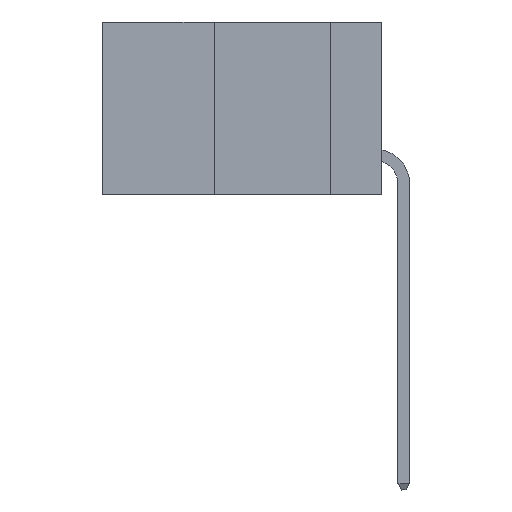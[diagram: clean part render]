
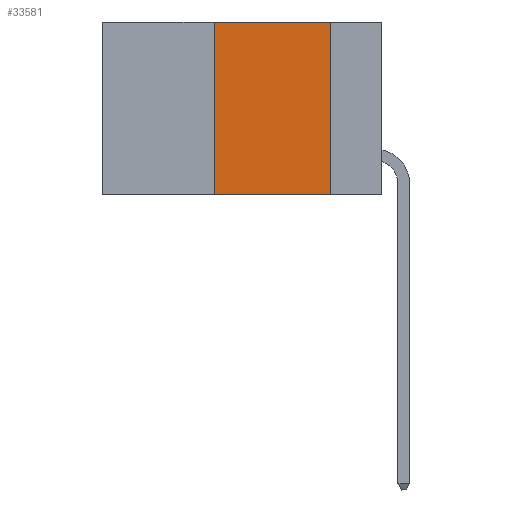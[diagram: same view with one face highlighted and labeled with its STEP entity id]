
A CAD part, left-side view. The second image highlights one B-rep face of the part: STEP entity #33581.
In plain terms, the highlighted planar face has unit normal (-1, 0, 0).
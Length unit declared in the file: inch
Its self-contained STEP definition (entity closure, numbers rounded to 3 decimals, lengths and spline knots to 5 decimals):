
#94 = VECTOR ( 'NONE', #6716, 39.37008 ) ;
#157 = VECTOR ( 'NONE', #35908, 39.37008 ) ;
#442 = ORIENTED_EDGE ( 'NONE', *, *, #18130, .F. ) ;
#4446 = ORIENTED_EDGE ( 'NONE', *, *, #7957, .T. ) ;
#4661 = EDGE_LOOP ( 'NONE', ( #442, #22245, #21265, #4446 ) ) ;
#6716 = DIRECTION ( 'NONE',  ( 0., 0., -1. ) ) ;
#7957 = EDGE_CURVE ( 'NONE', #26516, #17868, #40370, .T. ) ;
#8810 = PLANE ( 'NONE',  #37498 ) ;
#9765 = CARTESIAN_POINT ( 'NONE',  ( 0., 0.11, 0. ) ) ;
#10252 = EDGE_CURVE ( 'NONE', #26516, #10833, #16312, .T. ) ;
#10833 = VERTEX_POINT ( 'NONE', #28313 ) ;
#14839 = EDGE_CURVE ( 'NONE', #10833, #34850, #32149, .T. ) ;
#16312 = LINE ( 'NONE', #22886, #26755 ) ;
#16347 = DIRECTION ( 'NONE',  ( 0., 0., 1. ) ) ;
#16848 = CARTESIAN_POINT ( 'NONE',  ( 0., 0.6, 0. ) ) ;
#17218 = CARTESIAN_POINT ( 'NONE',  ( 0., 0.11, -0.37 ) ) ;
#17868 = VERTEX_POINT ( 'NONE', #17218 ) ;
#18130 = EDGE_CURVE ( 'NONE', #34850, #17868, #27435, .T. ) ;
#19181 = CARTESIAN_POINT ( 'NONE',  ( 0., 0.36, -0.37 ) ) ;
#21265 = ORIENTED_EDGE ( 'NONE', *, *, #10252, .F. ) ;
#21677 = DIRECTION ( 'NONE',  ( 0., 0., -1. ) ) ;
#22245 = ORIENTED_EDGE ( 'NONE', *, *, #14839, .F. ) ;
#22429 = FACE_OUTER_BOUND ( 'NONE', #4661, .T. ) ;
#22886 = CARTESIAN_POINT ( 'NONE',  ( 0., 0.36, 0. ) ) ;
#26516 = VERTEX_POINT ( 'NONE', #19181 ) ;
#26755 = VECTOR ( 'NONE', #16347, 39.37008 ) ;
#27435 = LINE ( 'NONE', #9765, #94 ) ;
#28313 = CARTESIAN_POINT ( 'NONE',  ( 0., 0.36, 0. ) ) ;
#29318 = DIRECTION ( 'NONE',  ( 0., -1., 0. ) ) ;
#31169 = VECTOR ( 'NONE', #29318, 39.37008 ) ;
#32149 = LINE ( 'NONE', #16848, #31169 ) ;
#32703 = CARTESIAN_POINT ( 'NONE',  ( 0., 0.6, -0.37 ) ) ;
#33581 = ADVANCED_FACE ( 'NONE', ( #22429 ), #8810, .F. ) ;
#34127 = CARTESIAN_POINT ( 'NONE',  ( 0., 0.6, 0. ) ) ;
#34850 = VERTEX_POINT ( 'NONE', #38366 ) ;
#35908 = DIRECTION ( 'NONE',  ( 0., -1., 0. ) ) ;
#37498 = AXIS2_PLACEMENT_3D ( 'NONE', #34127, #40620, #21677 ) ;
#38366 = CARTESIAN_POINT ( 'NONE',  ( 0., 0.11, 0. ) ) ;
#40370 = LINE ( 'NONE', #32703, #157 ) ;
#40620 = DIRECTION ( 'NONE',  ( 1., 0., 0. ) ) ;
